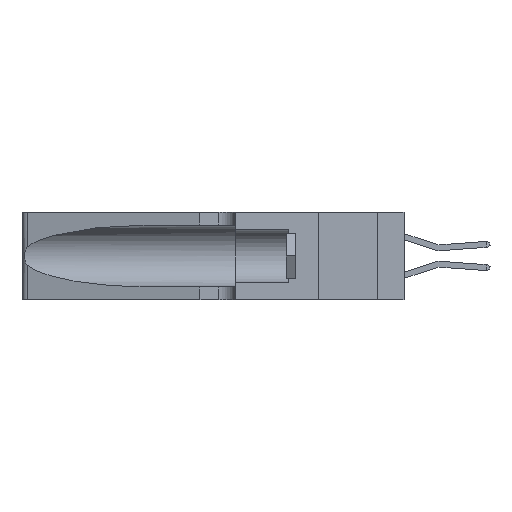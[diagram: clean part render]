
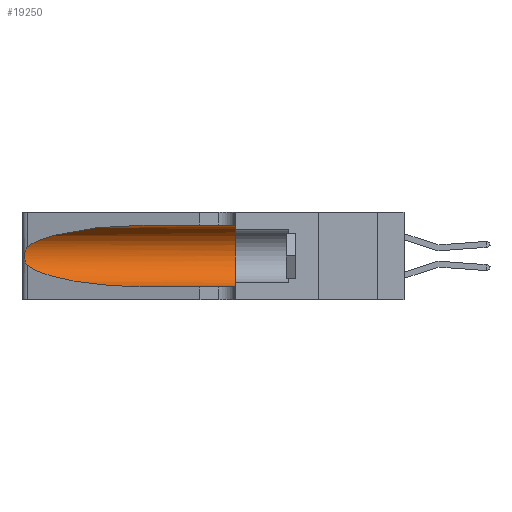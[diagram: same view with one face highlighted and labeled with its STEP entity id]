
A CAD part, left-side view. The second image highlights one B-rep face of the part: STEP entity #19250.
In plain terms, the highlighted cylindrical face has radius 3.308 mm (diameter 6.617 mm), a partial arc.
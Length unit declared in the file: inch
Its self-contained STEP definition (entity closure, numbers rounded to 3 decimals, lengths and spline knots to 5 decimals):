
#1520 =( BOUNDED_CURVE ( )  B_SPLINE_CURVE ( 3, ( #29323, #8859, #39055, #42603 ),
 .UNSPECIFIED., .F., .F. ) 
 B_SPLINE_CURVE_WITH_KNOTS ( ( 4, 4 ),
 ( 3.44316, 4.71239 ),
 .UNSPECIFIED. ) 
 CURVE ( )  GEOMETRIC_REPRESENTATION_ITEM ( )  RATIONAL_B_SPLINE_CURVE ( ( 1., 0.87, 0.87, 1. ) ) 
 REPRESENTATION_ITEM ( '' )  );
#1687 = AXIS2_PLACEMENT_3D ( 'NONE', #38846, #36139, #26046 ) ;
#1783 = CARTESIAN_POINT ( 'NONE',  ( 0.26017, 1.23833, 0.17102 ) ) ;
#2183 = VERTEX_POINT ( 'NONE', #15281 ) ;
#2720 = CARTESIAN_POINT ( 'NONE',  ( 0.1305, 0.35, 0.185 ) ) ;
#3338 = VERTEX_POINT ( 'NONE', #12088 ) ;
#4936 = VERTEX_POINT ( 'NONE', #38278 ) ;
#4970 = DIRECTION ( 'NONE',  ( 0., -1., 0. ) ) ;
#5063 = ORIENTED_EDGE ( 'NONE', *, *, #24810, .T. ) ;
#5299 = VECTOR ( 'NONE', #4970, 39.37008 ) ;
#5643 = CARTESIAN_POINT ( 'NONE',  ( 0.1305, 0.72297, 0.31525 ) ) ;
#5731 = CARTESIAN_POINT ( 'NONE',  ( 0.25639, 1.23186, 0.15144 ) ) ;
#6327 = EDGE_CURVE ( 'NONE', #15326, #4936, #1520, .T. ) ;
#6336 = CARTESIAN_POINT ( 'NONE',  ( 0.25487, 1.22718, 0.22369 ) ) ;
#7091 = ORIENTED_EDGE ( 'NONE', *, *, #28738, .T. ) ;
#7986 =( BOUNDED_CURVE ( )  B_SPLINE_CURVE ( 3, ( #5643, #12007, #25685, #6336 ),
 .UNSPECIFIED., .F., .T. ) 
 B_SPLINE_CURVE_WITH_KNOTS ( ( 4, 4 ),
 ( 1.5708, 2.84003 ),
 .UNSPECIFIED. ) 
 CURVE ( )  GEOMETRIC_REPRESENTATION_ITEM ( )  RATIONAL_B_SPLINE_CURVE ( ( 1., 0.87, 0.87, 1. ) ) 
 REPRESENTATION_ITEM ( '' )  );
#8062 = DIRECTION ( 'NONE',  ( 0., -1., 0. ) ) ;
#8391 = FACE_OUTER_BOUND ( 'NONE', #21004, .T. ) ;
#8859 = CARTESIAN_POINT ( 'NONE',  ( 0.2373, 1.15595, 0.08982 ) ) ;
#9503 = ORIENTED_EDGE ( 'NONE', *, *, #6327, .T. ) ;
#9862 = CARTESIAN_POINT ( 'NONE',  ( 0.25555, 1.22994, 0.2215 ) ) ;
#9958 = VERTEX_POINT ( 'NONE', #21646 ) ;
#10286 = CARTESIAN_POINT ( 'NONE',  ( 0.25487, 1.22718, 0.22369 ) ) ;
#12007 = CARTESIAN_POINT ( 'NONE',  ( 0.18966, 0.96281, 0.31525 ) ) ;
#12066 = EDGE_CURVE ( 'NONE', #9958, #2183, #23731, .T. ) ;
#12088 = CARTESIAN_POINT ( 'NONE',  ( 0.1305, 0.35, 0.05475 ) ) ;
#12623 = AXIS2_PLACEMENT_3D ( 'NONE', #2720, #19656, #29629 ) ;
#12683 = CARTESIAN_POINT ( 'NONE',  ( 0.25487, 1.22718, 0.14631 ) ) ;
#13318 = CARTESIAN_POINT ( 'NONE',  ( 0.25487, 1.22718, 0.22369 ) ) ;
#15183 = CARTESIAN_POINT ( 'NONE',  ( 0.25856, 1.23593, 0.16098 ) ) ;
#15281 = CARTESIAN_POINT ( 'NONE',  ( 0.1305, 0.35, 0.31525 ) ) ;
#15326 = VERTEX_POINT ( 'NONE', #26903 ) ;
#15760 = CARTESIAN_POINT ( 'NONE',  ( 0.26018, 1.23835, 0.19895 ) ) ;
#16745 = CARTESIAN_POINT ( 'NONE',  ( 0.25854, 1.2359, 0.20912 ) ) ;
#18209 = CARTESIAN_POINT ( 'NONE',  ( 0.1305, 1.61858, 0.31525 ) ) ;
#19023 = VECTOR ( 'NONE', #8062, 39.37008 ) ;
#19250 = ADVANCED_FACE ( 'NONE', ( #8391 ), #43364, .F. ) ;
#19543 = ORIENTED_EDGE ( 'NONE', *, *, #12066, .F. ) ;
#19614 = CARTESIAN_POINT ( 'NONE',  ( 0.25789, 1.23486, 0.15765 ) ) ;
#19656 = DIRECTION ( 'NONE',  ( 0., 1., 0. ) ) ;
#20963 = B_SPLINE_CURVE_WITH_KNOTS ( 'NONE', 3,
 ( #10286, #9862, #33161, #30593, #16745, #15760, #31585, #31877, #1783, #15183, #19614, #5731, #22974, #12683 ),
 .UNSPECIFIED., .F., .F.,
 ( 4, 2, 2, 2, 2, 2, 4 ),
 ( 0., 0.00027, 0.00053, 0.00107, 0.0016, 0.00187, 0.00214 ),
 .UNSPECIFIED. ) ;
#21004 = EDGE_LOOP ( 'NONE', ( #5063, #7091, #9503, #21199, #43780, #19543 ) ) ;
#21199 = ORIENTED_EDGE ( 'NONE', *, *, #34938, .T. ) ;
#21563 = VERTEX_POINT ( 'NONE', #13318 ) ;
#21646 = CARTESIAN_POINT ( 'NONE',  ( 0.1305, 0.72297, 0.31525 ) ) ;
#22974 = CARTESIAN_POINT ( 'NONE',  ( 0.25555, 1.22993, 0.14849 ) ) ;
#23731 = LINE ( 'NONE', #18209, #5299 ) ;
#24810 = EDGE_CURVE ( 'NONE', #9958, #21563, #7986, .T. ) ;
#25685 = CARTESIAN_POINT ( 'NONE',  ( 0.2373, 1.15595, 0.28018 ) ) ;
#26046 = DIRECTION ( 'NONE',  ( 0., 0., -1. ) ) ;
#26903 = CARTESIAN_POINT ( 'NONE',  ( 0.25487, 1.22718, 0.14631 ) ) ;
#27974 = CARTESIAN_POINT ( 'NONE',  ( 0.1305, 1.61858, 0.05475 ) ) ;
#28738 = EDGE_CURVE ( 'NONE', #21563, #15326, #20963, .T. ) ;
#29323 = CARTESIAN_POINT ( 'NONE',  ( 0.25487, 1.22718, 0.14631 ) ) ;
#29629 = DIRECTION ( 'NONE',  ( 0., 0., 1. ) ) ;
#30593 = CARTESIAN_POINT ( 'NONE',  ( 0.25787, 1.23484, 0.2124 ) ) ;
#31585 = CARTESIAN_POINT ( 'NONE',  ( 0.26075, 1.23896, 0.19203 ) ) ;
#31644 = CIRCLE ( 'NONE', #12623, 0.13025 ) ;
#31877 = CARTESIAN_POINT ( 'NONE',  ( 0.26075, 1.23896, 0.178 ) ) ;
#33161 = CARTESIAN_POINT ( 'NONE',  ( 0.25639, 1.23184, 0.21858 ) ) ;
#34938 = EDGE_CURVE ( 'NONE', #4936, #3338, #41259, .T. ) ;
#36139 = DIRECTION ( 'NONE',  ( 0., -1., 0. ) ) ;
#38278 = CARTESIAN_POINT ( 'NONE',  ( 0.1305, 0.72297, 0.05475 ) ) ;
#38846 = CARTESIAN_POINT ( 'NONE',  ( 0.1305, 1.61858, 0.185 ) ) ;
#39055 = CARTESIAN_POINT ( 'NONE',  ( 0.18966, 0.96281, 0.05475 ) ) ;
#41259 = LINE ( 'NONE', #27974, #19023 ) ;
#42603 = CARTESIAN_POINT ( 'NONE',  ( 0.1305, 0.72297, 0.05475 ) ) ;
#42968 = EDGE_CURVE ( 'NONE', #2183, #3338, #31644, .T. ) ;
#43364 = CYLINDRICAL_SURFACE ( 'NONE', #1687, 0.13025 ) ;
#43780 = ORIENTED_EDGE ( 'NONE', *, *, #42968, .F. ) ;
